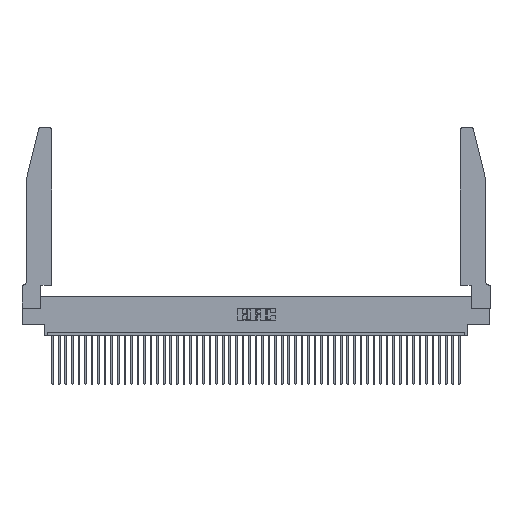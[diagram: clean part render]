
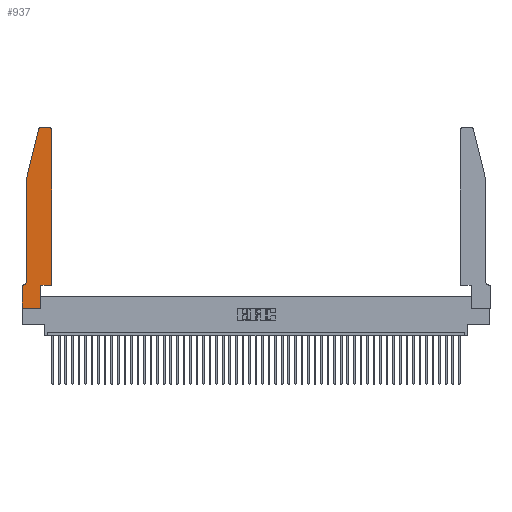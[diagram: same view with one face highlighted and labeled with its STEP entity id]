
A CAD part, top view. The second image highlights one B-rep face of the part: STEP entity #937.
In plain terms, the highlighted planar face has unit normal (0, 0, 1).
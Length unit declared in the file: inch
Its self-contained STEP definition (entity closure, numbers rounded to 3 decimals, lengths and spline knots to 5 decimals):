
#344 = ORIENTED_EDGE ( 'NONE', *, *, #39150, .T. ) ;
#937 = ADVANCED_FACE ( 'NONE', ( #30183 ), #44287, .T. ) ;
#1339 = VERTEX_POINT ( 'NONE', #5050 ) ;
#1566 = CARTESIAN_POINT ( 'NONE',  ( 0.25487, 2.72718, 0.37 ) ) ;
#1747 = DIRECTION ( 'NONE',  ( 0., 0., 1. ) ) ;
#1905 = VECTOR ( 'NONE', #46395, 39.37008 ) ;
#2461 = CARTESIAN_POINT ( 'NONE',  ( 0.284, 2.75, 0.37 ) ) ;
#4504 = CARTESIAN_POINT ( 'NONE',  ( 0.2865, 0., 0.37 ) ) ;
#4810 = DIRECTION ( 'NONE',  ( 0., 1., 0. ) ) ;
#5050 = CARTESIAN_POINT ( 'NONE',  ( 0.4205, 2.75, 0.37 ) ) ;
#5202 = DIRECTION ( 'NONE',  ( 0., 0., -1. ) ) ;
#5646 = CARTESIAN_POINT ( 'NONE',  ( 0., 0., 0.37 ) ) ;
#6258 = VERTEX_POINT ( 'NONE', #2461 ) ;
#7372 = EDGE_CURVE ( 'NONE', #30004, #1339, #32648, .T. ) ;
#7481 = VERTEX_POINT ( 'NONE', #4504 ) ;
#8610 = CARTESIAN_POINT ( 'NONE',  ( 0.4505, 0.35, 0.37 ) ) ;
#8834 = VECTOR ( 'NONE', #37333, 39.37008 ) ;
#9173 = DIRECTION ( 'NONE',  ( 0., 0., 1. ) ) ;
#9817 = CARTESIAN_POINT ( 'NONE',  ( 0.4505, 0.35, 0.37 ) ) ;
#9918 = VECTOR ( 'NONE', #35895, 39.37008 ) ;
#10356 = DIRECTION ( 'NONE',  ( 0., -1., 0. ) ) ;
#10998 = VERTEX_POINT ( 'NONE', #29610 ) ;
#11237 = AXIS2_PLACEMENT_3D ( 'NONE', #24662, #1747, #36533 ) ;
#11430 = VERTEX_POINT ( 'NONE', #1566 ) ;
#11754 = VERTEX_POINT ( 'NONE', #13739 ) ;
#12459 = DIRECTION ( 'NONE',  ( 0., 1., 0. ) ) ;
#12575 = EDGE_CURVE ( 'NONE', #7481, #42228, #39171, .T. ) ;
#13739 = CARTESIAN_POINT ( 'NONE',  ( 0.0055, 0.35, 0.37 ) ) ;
#16198 = VECTOR ( 'NONE', #47936, 39.37008 ) ;
#17047 = VERTEX_POINT ( 'NONE', #26726 ) ;
#17100 = CARTESIAN_POINT ( 'NONE',  ( 0.0055, 0.42, 0.37 ) ) ;
#17552 = ORIENTED_EDGE ( 'NONE', *, *, #45224, .T. ) ;
#17701 = CARTESIAN_POINT ( 'NONE',  ( 0.0755, 0.35, 0.37 ) ) ;
#18900 = VECTOR ( 'NONE', #10356, 39.37008 ) ;
#18919 = DIRECTION ( 'NONE',  ( 1., 0., 0. ) ) ;
#20059 = LINE ( 'NONE', #5646, #9918 ) ;
#20754 = DIRECTION ( 'NONE',  ( -1., 0., 0. ) ) ;
#20979 = AXIS2_PLACEMENT_3D ( 'NONE', #29055, #25560, #21861 ) ;
#21861 = DIRECTION ( 'NONE',  ( 1., 0., 0. ) ) ;
#21911 = ORIENTED_EDGE ( 'NONE', *, *, #7372, .T. ) ;
#23368 = ORIENTED_EDGE ( 'NONE', *, *, #29730, .T. ) ;
#24158 = ORIENTED_EDGE ( 'NONE', *, *, #42576, .T. ) ;
#24662 = CARTESIAN_POINT ( 'NONE',  ( 0.4205, 2.72, 0.37 ) ) ;
#25560 = DIRECTION ( 'NONE',  ( 0., 0., 1. ) ) ;
#26156 = CARTESIAN_POINT ( 'NONE',  ( 0., 0., 0.37 ) ) ;
#26236 = CARTESIAN_POINT ( 'NONE',  ( 0.2865, 0.35, 0.37 ) ) ;
#26582 = ORIENTED_EDGE ( 'NONE', *, *, #27258, .T. ) ;
#26726 = CARTESIAN_POINT ( 'NONE',  ( 0., 0., 0.37 ) ) ;
#26858 = LINE ( 'NONE', #36790, #8834 ) ;
#27258 = EDGE_CURVE ( 'NONE', #41523, #30004, #48071, .T. ) ;
#27703 = CIRCLE ( 'NONE', #27987, 0.03 ) ;
#27987 = AXIS2_PLACEMENT_3D ( 'NONE', #34976, #9173, #39640 ) ;
#28251 = LINE ( 'NONE', #42092, #1905 ) ;
#28837 = VECTOR ( 'NONE', #44471, 39.37008 ) ;
#29055 = CARTESIAN_POINT ( 'NONE',  ( 0., 0.35, 0.37 ) ) ;
#29431 = ORIENTED_EDGE ( 'NONE', *, *, #44680, .T. ) ;
#29610 = CARTESIAN_POINT ( 'NONE',  ( 0., 0.35, 0.37 ) ) ;
#29730 = EDGE_CURVE ( 'NONE', #11430, #33669, #26858, .T. ) ;
#29836 = CARTESIAN_POINT ( 'NONE',  ( 0.0755, 0.42, 0.37 ) ) ;
#30004 = VERTEX_POINT ( 'NONE', #34535 ) ;
#30183 = FACE_OUTER_BOUND ( 'NONE', #39594, .T. ) ;
#30840 = VERTEX_POINT ( 'NONE', #29836 ) ;
#30913 = CARTESIAN_POINT ( 'NONE',  ( 0.0755, 2., 0.37 ) ) ;
#31150 = EDGE_CURVE ( 'NONE', #10998, #17047, #20059, .T. ) ;
#32124 = EDGE_CURVE ( 'NONE', #33669, #30840, #36848, .T. ) ;
#32538 = CARTESIAN_POINT ( 'NONE',  ( 0.4505, 0.35, 0.37 ) ) ;
#32648 = CIRCLE ( 'NONE', #11237, 0.03 ) ;
#33669 = VERTEX_POINT ( 'NONE', #30913 ) ;
#33848 = VECTOR ( 'NONE', #4810, 39.37008 ) ;
#34535 = CARTESIAN_POINT ( 'NONE',  ( 0.4505, 2.72, 0.37 ) ) ;
#34976 = CARTESIAN_POINT ( 'NONE',  ( 0.284, 2.72, 0.37 ) ) ;
#35849 = ORIENTED_EDGE ( 'NONE', *, *, #44979, .T. ) ;
#35895 = DIRECTION ( 'NONE',  ( 0., -1., 0. ) ) ;
#35930 = ORIENTED_EDGE ( 'NONE', *, *, #12575, .T. ) ;
#35988 = LINE ( 'NONE', #17701, #28837 ) ;
#36533 = DIRECTION ( 'NONE',  ( 1., 0., 0. ) ) ;
#36790 = CARTESIAN_POINT ( 'NONE',  ( 0.0755, 2., 0.37 ) ) ;
#36848 = LINE ( 'NONE', #42483, #18900 ) ;
#37301 = VECTOR ( 'NONE', #12459, 39.37008 ) ;
#37333 = DIRECTION ( 'NONE',  ( -0.239, -0.971, 0. ) ) ;
#37514 = ORIENTED_EDGE ( 'NONE', *, *, #32124, .T. ) ;
#39150 = EDGE_CURVE ( 'NONE', #6258, #11430, #27703, .T. ) ;
#39171 = LINE ( 'NONE', #43634, #33848 ) ;
#39594 = EDGE_LOOP ( 'NONE', ( #35849, #344, #23368, #37514, #24158, #29431, #42235, #40320, #35930, #17552, #26582, #21911 ) ) ;
#39640 = DIRECTION ( 'NONE',  ( 1., 0., 0. ) ) ;
#39656 = LINE ( 'NONE', #26156, #44490 ) ;
#40320 = ORIENTED_EDGE ( 'NONE', *, *, #44143, .T. ) ;
#40517 = CIRCLE ( 'NONE', #44794, 0.07 ) ;
#41523 = VERTEX_POINT ( 'NONE', #9817 ) ;
#42092 = CARTESIAN_POINT ( 'NONE',  ( 0.2605, 2.75, 0.37 ) ) ;
#42228 = VERTEX_POINT ( 'NONE', #26236 ) ;
#42235 = ORIENTED_EDGE ( 'NONE', *, *, #31150, .T. ) ;
#42483 = CARTESIAN_POINT ( 'NONE',  ( 0.0755, 2., 0.37 ) ) ;
#42576 = EDGE_CURVE ( 'NONE', #30840, #11754, #40517, .T. ) ;
#43634 = CARTESIAN_POINT ( 'NONE',  ( 0.2865, 0.35, 0.37 ) ) ;
#44143 = EDGE_CURVE ( 'NONE', #17047, #7481, #39656, .T. ) ;
#44287 = PLANE ( 'NONE',  #20979 ) ;
#44471 = DIRECTION ( 'NONE',  ( -1., 0., 0. ) ) ;
#44490 = VECTOR ( 'NONE', #18919, 39.37008 ) ;
#44680 = EDGE_CURVE ( 'NONE', #11754, #10998, #35988, .T. ) ;
#44794 = AXIS2_PLACEMENT_3D ( 'NONE', #17100, #5202, #20754 ) ;
#44979 = EDGE_CURVE ( 'NONE', #1339, #6258, #28251, .T. ) ;
#45004 = LINE ( 'NONE', #32538, #16198 ) ;
#45224 = EDGE_CURVE ( 'NONE', #42228, #41523, #45004, .T. ) ;
#46395 = DIRECTION ( 'NONE',  ( -1., 0., 0. ) ) ;
#47936 = DIRECTION ( 'NONE',  ( 1., 0., 0. ) ) ;
#48071 = LINE ( 'NONE', #8610, #37301 ) ;
